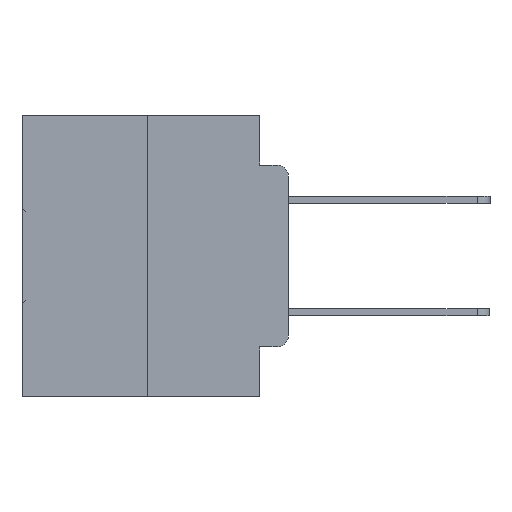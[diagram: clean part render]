
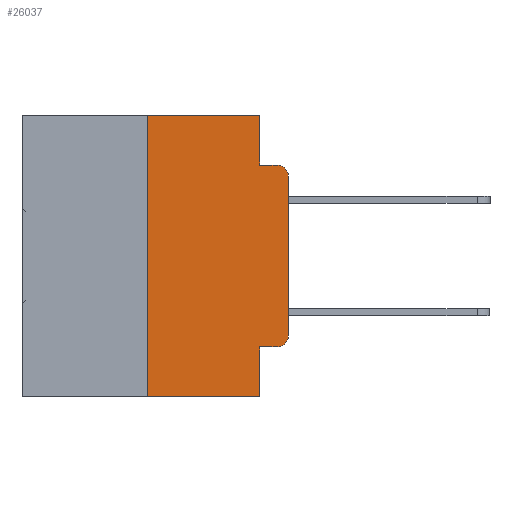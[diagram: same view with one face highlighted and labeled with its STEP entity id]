
A CAD part, left-side view. The second image highlights one B-rep face of the part: STEP entity #26037.
In plain terms, the highlighted planar face has unit normal (-1, 0, 0).
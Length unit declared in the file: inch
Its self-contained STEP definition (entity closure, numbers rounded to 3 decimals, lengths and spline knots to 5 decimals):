
#182 = LINE ( 'NONE', #31373, #7113 ) ;
#544 = ORIENTED_EDGE ( 'NONE', *, *, #16230, .F. ) ;
#651 = DIRECTION ( 'NONE',  ( 0., 0., 1. ) ) ;
#1000 = ORIENTED_EDGE ( 'NONE', *, *, #32122, .T. ) ;
#1054 = VERTEX_POINT ( 'NONE', #7026 ) ;
#1674 = VECTOR ( 'NONE', #3364, 39.37008 ) ;
#1807 = ORIENTED_EDGE ( 'NONE', *, *, #20349, .F. ) ;
#1839 = AXIS2_PLACEMENT_3D ( 'NONE', #11874, #29627, #14471 ) ;
#2079 = LINE ( 'NONE', #16625, #15056 ) ;
#2297 = PLANE ( 'NONE',  #31068 ) ;
#3364 = DIRECTION ( 'NONE',  ( 0., 0., -1. ) ) ;
#3637 = CARTESIAN_POINT ( 'NONE',  ( 0., 0.25, -0.5 ) ) ;
#4365 = CIRCLE ( 'NONE', #6417, 0.02 ) ;
#4376 = VERTEX_POINT ( 'NONE', #5242 ) ;
#5242 = CARTESIAN_POINT ( 'NONE',  ( 0., 0.051, -0.5 ) ) ;
#5801 = CARTESIAN_POINT ( 'NONE',  ( 0., 0.051, -0.0885 ) ) ;
#6145 = CARTESIAN_POINT ( 'NONE',  ( 0., 0.25, 0. ) ) ;
#6417 = AXIS2_PLACEMENT_3D ( 'NONE', #26047, #10779, #28596 ) ;
#7026 = CARTESIAN_POINT ( 'NONE',  ( 0., 0.051, -0.4115 ) ) ;
#7044 = ORIENTED_EDGE ( 'NONE', *, *, #19334, .T. ) ;
#7113 = VECTOR ( 'NONE', #651, 39.37008 ) ;
#7276 = CARTESIAN_POINT ( 'NONE',  ( 0., 0., 0. ) ) ;
#7497 = ORIENTED_EDGE ( 'NONE', *, *, #7698, .T. ) ;
#7698 = EDGE_CURVE ( 'NONE', #13361, #4376, #21618, .T. ) ;
#7854 = ORIENTED_EDGE ( 'NONE', *, *, #19388, .F. ) ;
#8106 = LINE ( 'NONE', #7276, #26872 ) ;
#8409 = DIRECTION ( 'NONE',  ( 0., -1., 0. ) ) ;
#8526 = CIRCLE ( 'NONE', #1839, 0.02 ) ;
#8611 = CARTESIAN_POINT ( 'NONE',  ( 0., 0.473, 0. ) ) ;
#9888 = DIRECTION ( 'NONE',  ( 0., 0., 1. ) ) ;
#10779 = DIRECTION ( 'NONE',  ( -1., 0., 0. ) ) ;
#10927 = CARTESIAN_POINT ( 'NONE',  ( 0., 0.02, -0.0885 ) ) ;
#11210 = DIRECTION ( 'NONE',  ( 0., -1., 0. ) ) ;
#11285 = CARTESIAN_POINT ( 'NONE',  ( 0., 0.02, -0.4115 ) ) ;
#11409 = LINE ( 'NONE', #19273, #24173 ) ;
#11874 = CARTESIAN_POINT ( 'NONE',  ( 0., 0.02, -0.3915 ) ) ;
#12052 = EDGE_CURVE ( 'NONE', #1054, #4376, #2079, .T. ) ;
#13361 = VERTEX_POINT ( 'NONE', #3637 ) ;
#14471 = DIRECTION ( 'NONE',  ( 0., 0., -1. ) ) ;
#14867 = VECTOR ( 'NONE', #27019, 39.37008 ) ;
#15056 = VECTOR ( 'NONE', #19173, 39.37008 ) ;
#15202 = ORIENTED_EDGE ( 'NONE', *, *, #12052, .F. ) ;
#16230 = EDGE_CURVE ( 'NONE', #25113, #18425, #28110, .T. ) ;
#16309 = VERTEX_POINT ( 'NONE', #11285 ) ;
#16365 = EDGE_CURVE ( 'NONE', #1054, #16309, #11409, .T. ) ;
#16625 = CARTESIAN_POINT ( 'NONE',  ( 0., 0.051, 0. ) ) ;
#16721 = DIRECTION ( 'NONE',  ( 0., -1., 0. ) ) ;
#18425 = VERTEX_POINT ( 'NONE', #22158 ) ;
#19173 = DIRECTION ( 'NONE',  ( 0., 0., -1. ) ) ;
#19273 = CARTESIAN_POINT ( 'NONE',  ( 0., 0.051, -0.4115 ) ) ;
#19334 = EDGE_CURVE ( 'NONE', #26073, #23852, #4365, .T. ) ;
#19388 = EDGE_CURVE ( 'NONE', #18425, #23852, #29148, .T. ) ;
#20249 = CARTESIAN_POINT ( 'NONE',  ( 0., 0.473, 0. ) ) ;
#20349 = EDGE_CURVE ( 'NONE', #13361, #28716, #182, .T. ) ;
#20356 = DIRECTION ( 'NONE',  ( 1., 0., 0. ) ) ;
#20375 = EDGE_CURVE ( 'NONE', #28716, #25113, #26699, .T. ) ;
#20494 = DIRECTION ( 'NONE',  ( 0., 0., -1. ) ) ;
#21618 = LINE ( 'NONE', #24490, #14867 ) ;
#21906 = ORIENTED_EDGE ( 'NONE', *, *, #32886, .T. ) ;
#22158 = CARTESIAN_POINT ( 'NONE',  ( 0., 0.051, -0.0885 ) ) ;
#22252 = VERTEX_POINT ( 'NONE', #23822 ) ;
#23237 = CARTESIAN_POINT ( 'NONE',  ( 0., 0., -0.1085 ) ) ;
#23238 = VECTOR ( 'NONE', #8409, 39.37008 ) ;
#23822 = CARTESIAN_POINT ( 'NONE',  ( 0., 0., -0.3915 ) ) ;
#23852 = VERTEX_POINT ( 'NONE', #10927 ) ;
#24173 = VECTOR ( 'NONE', #16721, 39.37008 ) ;
#24490 = CARTESIAN_POINT ( 'NONE',  ( 0., 0.473, -0.5 ) ) ;
#25113 = VERTEX_POINT ( 'NONE', #31466 ) ;
#26037 = ADVANCED_FACE ( 'NONE', ( #30396 ), #2297, .F. ) ;
#26047 = CARTESIAN_POINT ( 'NONE',  ( 0., 0.02, -0.1085 ) ) ;
#26073 = VERTEX_POINT ( 'NONE', #23237 ) ;
#26699 = LINE ( 'NONE', #8611, #32563 ) ;
#26872 = VECTOR ( 'NONE', #9888, 39.37008 ) ;
#27019 = DIRECTION ( 'NONE',  ( 0., -1., 0. ) ) ;
#27216 = EDGE_LOOP ( 'NONE', ( #21906, #7044, #7854, #544, #28629, #1807, #7497, #15202, #32556, #1000 ) ) ;
#28110 = LINE ( 'NONE', #28854, #1674 ) ;
#28596 = DIRECTION ( 'NONE',  ( 0., 0., -1. ) ) ;
#28629 = ORIENTED_EDGE ( 'NONE', *, *, #20375, .F. ) ;
#28716 = VERTEX_POINT ( 'NONE', #6145 ) ;
#28854 = CARTESIAN_POINT ( 'NONE',  ( 0., 0.051, 0. ) ) ;
#29148 = LINE ( 'NONE', #5801, #23238 ) ;
#29627 = DIRECTION ( 'NONE',  ( -1., 0., 0. ) ) ;
#30396 = FACE_OUTER_BOUND ( 'NONE', #27216, .T. ) ;
#31068 = AXIS2_PLACEMENT_3D ( 'NONE', #20249, #20356, #20494 ) ;
#31373 = CARTESIAN_POINT ( 'NONE',  ( 0., 0.25, 0. ) ) ;
#31466 = CARTESIAN_POINT ( 'NONE',  ( 0., 0.051, 0. ) ) ;
#32122 = EDGE_CURVE ( 'NONE', #16309, #22252, #8526, .T. ) ;
#32556 = ORIENTED_EDGE ( 'NONE', *, *, #16365, .T. ) ;
#32563 = VECTOR ( 'NONE', #11210, 39.37008 ) ;
#32886 = EDGE_CURVE ( 'NONE', #22252, #26073, #8106, .T. ) ;
